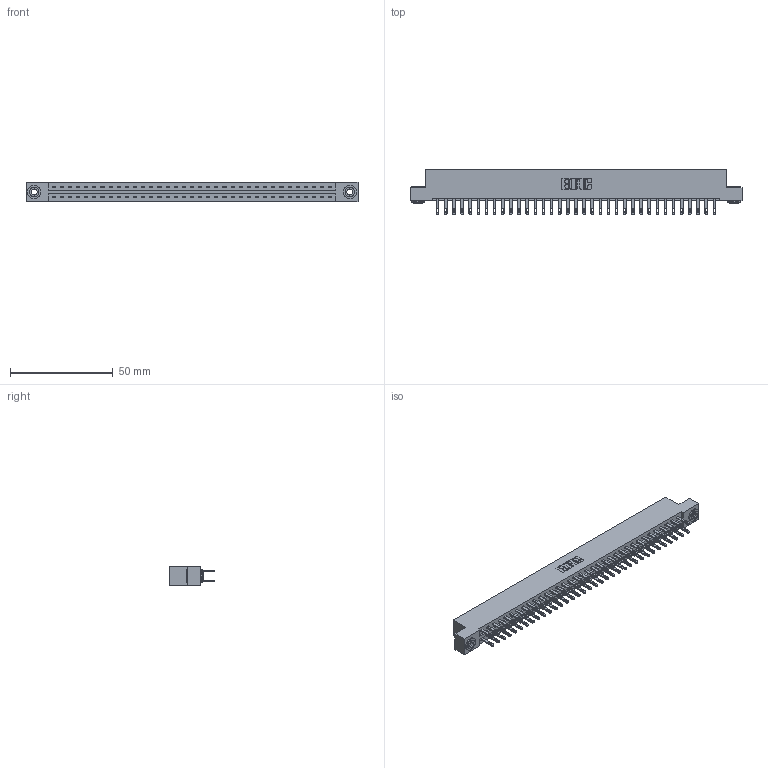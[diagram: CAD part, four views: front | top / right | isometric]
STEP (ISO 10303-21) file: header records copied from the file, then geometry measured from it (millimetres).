
FILE_DESCRIPTION (( 'STEP AP203' ), '1' );
FILE_NAME ('887-070-500-203.STEP', '2020-09-21T03:09:54', ( '' ), ( '' ), 'SwSTEP 2.0', 'SolidWorks 2020', '' );
FILE_SCHEMA (( 'CONFIG_CONTROL_DESIGN' ));
Length unit declared in the file: inch
Products named in the file (4): 345-250-002_345-250-002-102; 837 Part_Flush Mounting Lugs - 0.156 Dia-TH; 345-292-001_345-293-100; 887-070-500-203
Assembly tree (73 placements, depth 2):
  887-070-500-203
    837 Part_Flush Mounting Lugs - 0.156 Dia-TH
    345-292-001_345-293-100  x70
    345-250-002_345-250-002-102  x2
Bounding box: 161.7 x 21.85 x 9.4 mm (x, y, z)
Volume: 17181 mm3; surface area: 20356.2 mm2
Topology: 73 solids, 73 shells, 3652 faces, 11097 edges, 7394 vertices
Faces by surface type: plane 2320, cylinder 1324, cone 8
Entity records: 28622 total; most frequent: CARTESIAN_POINT 4801, ORIENTED_EDGE 4730, DIRECTION 4131, EDGE_CURVE 2365, LINE 2209, VECTOR 2209, VERTEX_POINT 1574, AXIS2_PLACEMENT_3D 961
